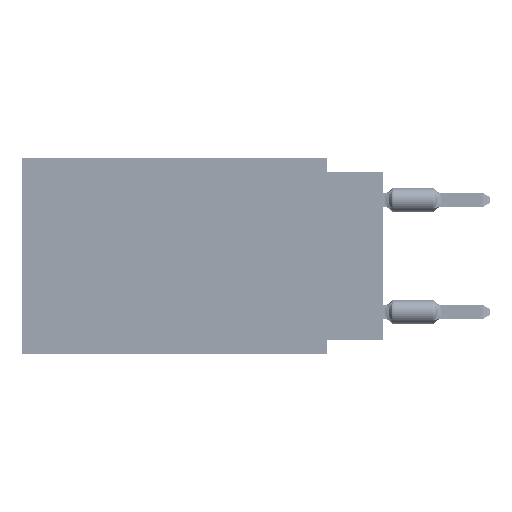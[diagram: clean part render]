
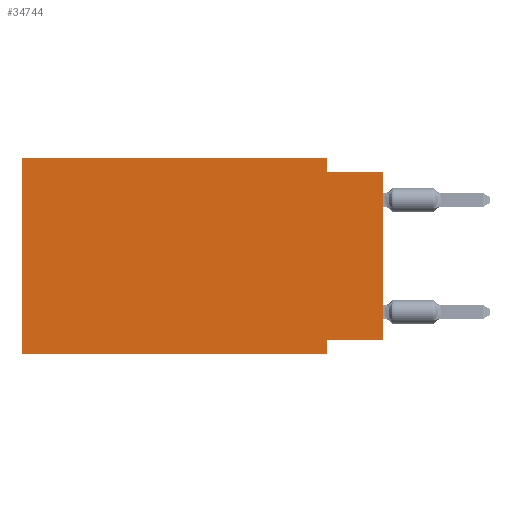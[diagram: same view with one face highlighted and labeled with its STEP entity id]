
A CAD part, left-side view. The second image highlights one B-rep face of the part: STEP entity #34744.
In plain terms, the highlighted planar face has unit normal (-1, 0, 0).
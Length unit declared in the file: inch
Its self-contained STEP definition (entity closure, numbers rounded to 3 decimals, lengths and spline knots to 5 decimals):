
#923 = CARTESIAN_POINT ( 'NONE',  ( 0., 0., -0.325 ) ) ;
#1240 = DIRECTION ( 'NONE',  ( 0., 1., 0. ) ) ;
#2310 = VERTEX_POINT ( 'NONE', #53945 ) ;
#4270 = EDGE_CURVE ( 'NONE', #2310, #40710, #21683, .T. ) ;
#5670 = LINE ( 'NONE', #46469, #23245 ) ;
#6022 = ORIENTED_EDGE ( 'NONE', *, *, #4270, .F. ) ;
#6646 = CARTESIAN_POINT ( 'NONE',  ( 0., 0.1, 0. ) ) ;
#7225 = CARTESIAN_POINT ( 'NONE',  ( 0., 0.1, -0.025 ) ) ;
#8324 = AXIS2_PLACEMENT_3D ( 'NONE', #31629, #21887, #52683 ) ;
#9854 = EDGE_CURVE ( 'NONE', #58114, #48975, #22911, .T. ) ;
#11019 = DIRECTION ( 'NONE',  ( 0., -1., 0. ) ) ;
#11328 = VECTOR ( 'NONE', #1240, 39.37008 ) ;
#11987 = ORIENTED_EDGE ( 'NONE', *, *, #39909, .F. ) ;
#13998 = DIRECTION ( 'NONE',  ( 0., -1., 0. ) ) ;
#14344 = CARTESIAN_POINT ( 'NONE',  ( 0., 0., 0. ) ) ;
#15038 = CARTESIAN_POINT ( 'NONE',  ( 0., 0.1, -0.325 ) ) ;
#16673 = DIRECTION ( 'NONE',  ( 0., -1., 0. ) ) ;
#17936 = VECTOR ( 'NONE', #19354, 39.37008 ) ;
#19354 = DIRECTION ( 'NONE',  ( 0., 0., 1. ) ) ;
#20620 = LINE ( 'NONE', #923, #11328 ) ;
#20780 = VERTEX_POINT ( 'NONE', #44793 ) ;
#21683 = LINE ( 'NONE', #6646, #43887 ) ;
#21887 = DIRECTION ( 'NONE',  ( 1., 0., 0. ) ) ;
#22544 = PLANE ( 'NONE',  #8324 ) ;
#22911 = LINE ( 'NONE', #14344, #17936 ) ;
#23245 = VECTOR ( 'NONE', #11019, 39.37008 ) ;
#25720 = CARTESIAN_POINT ( 'NONE',  ( 0., 0., -0.025 ) ) ;
#26848 = CARTESIAN_POINT ( 'NONE',  ( 0., 0., -0.325 ) ) ;
#29034 = DIRECTION ( 'NONE',  ( 0., 0., 1. ) ) ;
#31629 = CARTESIAN_POINT ( 'NONE',  ( 0., 0.645, 0. ) ) ;
#32585 = CARTESIAN_POINT ( 'NONE',  ( 0., 0.1, -0.35 ) ) ;
#32927 = FACE_OUTER_BOUND ( 'NONE', #59105, .T. ) ;
#33943 = VECTOR ( 'NONE', #34538, 39.37008 ) ;
#34538 = DIRECTION ( 'NONE',  ( 0., 0., -1. ) ) ;
#34744 = ADVANCED_FACE ( 'NONE', ( #32927 ), #22544, .F. ) ;
#35933 = ORIENTED_EDGE ( 'NONE', *, *, #42630, .F. ) ;
#37242 = VECTOR ( 'NONE', #13998, 39.37008 ) ;
#37776 = EDGE_CURVE ( 'NONE', #20780, #2310, #62170, .T. ) ;
#38433 = EDGE_CURVE ( 'NONE', #40710, #48975, #5670, .T. ) ;
#38748 = LINE ( 'NONE', #59148, #37242 ) ;
#38883 = LINE ( 'NONE', #49591, #33943 ) ;
#39909 = EDGE_CURVE ( 'NONE', #42347, #64526, #38883, .T. ) ;
#40710 = VERTEX_POINT ( 'NONE', #7225 ) ;
#42347 = VERTEX_POINT ( 'NONE', #15038 ) ;
#42630 = EDGE_CURVE ( 'NONE', #61176, #20780, #43427, .T. ) ;
#43427 = LINE ( 'NONE', #53471, #57956 ) ;
#43673 = ORIENTED_EDGE ( 'NONE', *, *, #38433, .F. ) ;
#43887 = VECTOR ( 'NONE', #62161, 39.37008 ) ;
#44599 = VECTOR ( 'NONE', #16673, 39.37008 ) ;
#44793 = CARTESIAN_POINT ( 'NONE',  ( 0., 0.645, 0. ) ) ;
#46384 = EDGE_CURVE ( 'NONE', #58114, #42347, #20620, .T. ) ;
#46469 = CARTESIAN_POINT ( 'NONE',  ( 0., 0., -0.025 ) ) ;
#48189 = CARTESIAN_POINT ( 'NONE',  ( 0., 0.645, -0.35 ) ) ;
#48975 = VERTEX_POINT ( 'NONE', #25720 ) ;
#49591 = CARTESIAN_POINT ( 'NONE',  ( 0., 0.1, -0.35 ) ) ;
#50295 = ORIENTED_EDGE ( 'NONE', *, *, #58786, .T. ) ;
#50884 = ORIENTED_EDGE ( 'NONE', *, *, #46384, .F. ) ;
#51497 = ORIENTED_EDGE ( 'NONE', *, *, #9854, .T. ) ;
#52488 = CARTESIAN_POINT ( 'NONE',  ( 0., 0.645, 0. ) ) ;
#52683 = DIRECTION ( 'NONE',  ( 0., 0., -1. ) ) ;
#53471 = CARTESIAN_POINT ( 'NONE',  ( 0., 0.645, 0. ) ) ;
#53945 = CARTESIAN_POINT ( 'NONE',  ( 0., 0.1, 0. ) ) ;
#54919 = ORIENTED_EDGE ( 'NONE', *, *, #37776, .F. ) ;
#57956 = VECTOR ( 'NONE', #29034, 39.37008 ) ;
#58114 = VERTEX_POINT ( 'NONE', #26848 ) ;
#58786 = EDGE_CURVE ( 'NONE', #61176, #64526, #38748, .T. ) ;
#59105 = EDGE_LOOP ( 'NONE', ( #51497, #43673, #6022, #54919, #35933, #50295, #11987, #50884 ) ) ;
#59148 = CARTESIAN_POINT ( 'NONE',  ( 0., 0.645, -0.35 ) ) ;
#61176 = VERTEX_POINT ( 'NONE', #48189 ) ;
#62161 = DIRECTION ( 'NONE',  ( 0., 0., -1. ) ) ;
#62170 = LINE ( 'NONE', #52488, #44599 ) ;
#64526 = VERTEX_POINT ( 'NONE', #32585 ) ;
